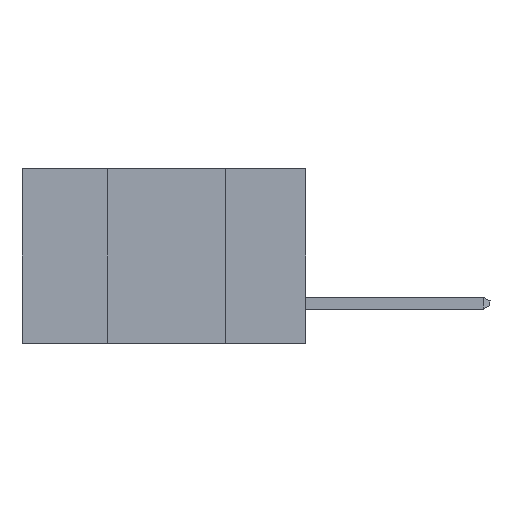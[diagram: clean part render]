
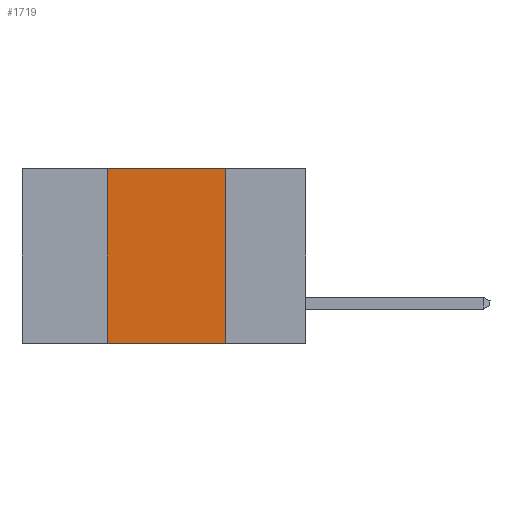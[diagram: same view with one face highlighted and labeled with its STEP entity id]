
A CAD part, left-side view. The second image highlights one B-rep face of the part: STEP entity #1719.
In plain terms, the highlighted planar face has unit normal (-1, 0, 0).
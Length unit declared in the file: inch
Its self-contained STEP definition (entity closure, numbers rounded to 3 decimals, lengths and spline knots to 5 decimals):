
#153 = PLANE ( 'NONE',  #1218 ) ;
#603 = CARTESIAN_POINT ( 'NONE',  ( 0., 0.6, -0.37 ) ) ;
#1218 = AXIS2_PLACEMENT_3D ( 'NONE', #8199, #15669, #12392 ) ;
#1719 = ADVANCED_FACE ( 'NONE', ( #18484 ), #153, .F. ) ;
#1834 = ORIENTED_EDGE ( 'NONE', *, *, #7670, .T. ) ;
#2032 = DIRECTION ( 'NONE',  ( 0., -1., 0. ) ) ;
#2072 = CARTESIAN_POINT ( 'NONE',  ( 0., 0.17, -0.37 ) ) ;
#2176 = ORIENTED_EDGE ( 'NONE', *, *, #15058, .F. ) ;
#3539 = ORIENTED_EDGE ( 'NONE', *, *, #12217, .F. ) ;
#3690 = DIRECTION ( 'NONE',  ( 0., 0., -1. ) ) ;
#3865 = VERTEX_POINT ( 'NONE', #14623 ) ;
#3869 = VECTOR ( 'NONE', #2032, 39.37008 ) ;
#4343 = VERTEX_POINT ( 'NONE', #13121 ) ;
#4365 = EDGE_LOOP ( 'NONE', ( #3539, #2176, #12663, #1834 ) ) ;
#4792 = LINE ( 'NONE', #18200, #11949 ) ;
#5690 = CARTESIAN_POINT ( 'NONE',  ( 0., 0.42, -0.37 ) ) ;
#6675 = LINE ( 'NONE', #2072, #13451 ) ;
#7045 = CARTESIAN_POINT ( 'NONE',  ( 0., 0.17, -0.37 ) ) ;
#7670 = EDGE_CURVE ( 'NONE', #3865, #11446, #15723, .T. ) ;
#8199 = CARTESIAN_POINT ( 'NONE',  ( 0., 0.6, 0. ) ) ;
#9979 = DIRECTION ( 'NONE',  ( 0., 0., 1. ) ) ;
#11446 = VERTEX_POINT ( 'NONE', #7045 ) ;
#11949 = VECTOR ( 'NONE', #15190, 39.37008 ) ;
#12217 = EDGE_CURVE ( 'NONE', #18753, #11446, #6675, .T. ) ;
#12263 = VECTOR ( 'NONE', #9979, 39.37008 ) ;
#12392 = DIRECTION ( 'NONE',  ( 0., 0., -1. ) ) ;
#12663 = ORIENTED_EDGE ( 'NONE', *, *, #15358, .F. ) ;
#13121 = CARTESIAN_POINT ( 'NONE',  ( 0., 0.42, 0. ) ) ;
#13285 = LINE ( 'NONE', #5690, #12263 ) ;
#13451 = VECTOR ( 'NONE', #3690, 39.37008 ) ;
#13636 = CARTESIAN_POINT ( 'NONE',  ( 0., 0.17, 0. ) ) ;
#14623 = CARTESIAN_POINT ( 'NONE',  ( 0., 0.42, -0.37 ) ) ;
#15058 = EDGE_CURVE ( 'NONE', #4343, #18753, #4792, .T. ) ;
#15190 = DIRECTION ( 'NONE',  ( 0., -1., 0. ) ) ;
#15358 = EDGE_CURVE ( 'NONE', #3865, #4343, #13285, .T. ) ;
#15669 = DIRECTION ( 'NONE',  ( 1., 0., 0. ) ) ;
#15723 = LINE ( 'NONE', #603, #3869 ) ;
#18200 = CARTESIAN_POINT ( 'NONE',  ( 0., 0.6, 0. ) ) ;
#18484 = FACE_OUTER_BOUND ( 'NONE', #4365, .T. ) ;
#18753 = VERTEX_POINT ( 'NONE', #13636 ) ;
